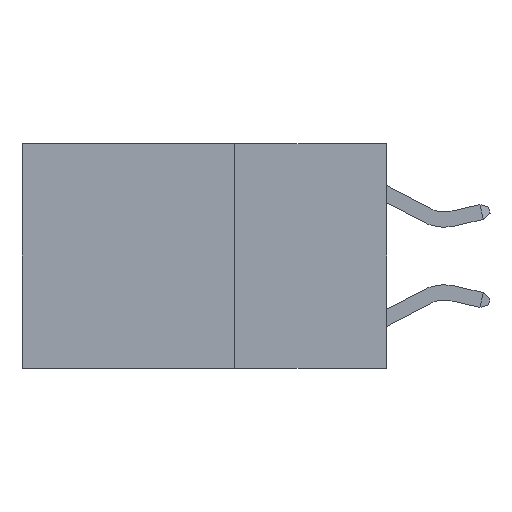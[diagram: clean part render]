
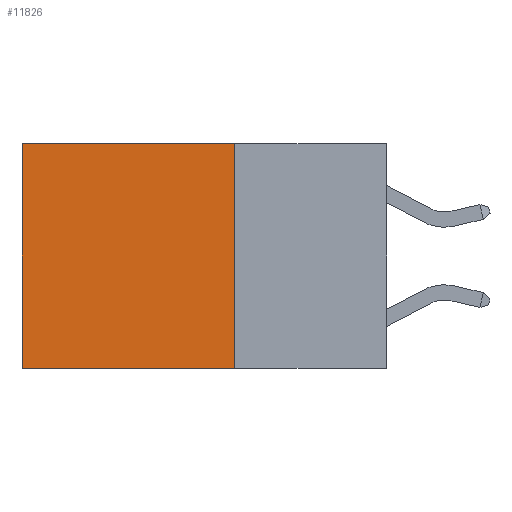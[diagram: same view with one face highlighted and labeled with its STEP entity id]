
A CAD part, left-side view. The second image highlights one B-rep face of the part: STEP entity #11826.
In plain terms, the highlighted planar face has unit normal (-1, 0, 0).
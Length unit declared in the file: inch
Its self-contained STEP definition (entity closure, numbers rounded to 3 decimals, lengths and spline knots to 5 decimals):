
#367 = VECTOR ( 'NONE', #10059, 39.37008 ) ;
#1426 = CARTESIAN_POINT ( 'NONE',  ( 0.2625, 0.25, -0.37 ) ) ;
#1536 = LINE ( 'NONE', #1426, #367 ) ;
#2218 = DIRECTION ( 'NONE',  ( 1., 0., 0. ) ) ;
#2482 = EDGE_CURVE ( 'NONE', #7998, #12967, #1536, .T. ) ;
#2577 = LINE ( 'NONE', #7992, #11697 ) ;
#3062 = FACE_OUTER_BOUND ( 'NONE', #7235, .T. ) ;
#3625 = CARTESIAN_POINT ( 'NONE',  ( 0.2625, 0.25, 0. ) ) ;
#4370 = VERTEX_POINT ( 'NONE', #8994 ) ;
#4670 = ORIENTED_EDGE ( 'NONE', *, *, #5070, .F. ) ;
#5047 = EDGE_CURVE ( 'NONE', #4370, #9518, #8269, .T. ) ;
#5070 = EDGE_CURVE ( 'NONE', #4370, #7998, #2577, .T. ) ;
#5331 = LINE ( 'NONE', #12869, #15397 ) ;
#5552 = DIRECTION ( 'NONE',  ( 0., 0., -1. ) ) ;
#7206 = PLANE ( 'NONE',  #10110 ) ;
#7235 = EDGE_LOOP ( 'NONE', ( #14538, #11356, #4670, #15577 ) ) ;
#7992 = CARTESIAN_POINT ( 'NONE',  ( 0.2625, 0.25, 0. ) ) ;
#7998 = VERTEX_POINT ( 'NONE', #10356 ) ;
#8269 = LINE ( 'NONE', #13014, #9039 ) ;
#8554 = CARTESIAN_POINT ( 'NONE',  ( 0.2625, 0.6, 0. ) ) ;
#8994 = CARTESIAN_POINT ( 'NONE',  ( 0.2625, 0.25, 0. ) ) ;
#9039 = VECTOR ( 'NONE', #15235, 39.37008 ) ;
#9518 = VERTEX_POINT ( 'NONE', #8554 ) ;
#10059 = DIRECTION ( 'NONE',  ( 0., 1., 0. ) ) ;
#10110 = AXIS2_PLACEMENT_3D ( 'NONE', #3625, #2218, #10727 ) ;
#10356 = CARTESIAN_POINT ( 'NONE',  ( 0.2625, 0.25, -0.37 ) ) ;
#10727 = DIRECTION ( 'NONE',  ( 0., 0., -1. ) ) ;
#11356 = ORIENTED_EDGE ( 'NONE', *, *, #2482, .F. ) ;
#11697 = VECTOR ( 'NONE', #13225, 39.37008 ) ;
#11826 = ADVANCED_FACE ( 'NONE', ( #3062 ), #7206, .F. ) ;
#12869 = CARTESIAN_POINT ( 'NONE',  ( 0.2625, 0.6, 0. ) ) ;
#12967 = VERTEX_POINT ( 'NONE', #14759 ) ;
#13014 = CARTESIAN_POINT ( 'NONE',  ( 0.2625, 0.25, 0. ) ) ;
#13225 = DIRECTION ( 'NONE',  ( 0., 0., -1. ) ) ;
#14538 = ORIENTED_EDGE ( 'NONE', *, *, #15135, .T. ) ;
#14759 = CARTESIAN_POINT ( 'NONE',  ( 0.2625, 0.6, -0.37 ) ) ;
#15135 = EDGE_CURVE ( 'NONE', #9518, #12967, #5331, .T. ) ;
#15235 = DIRECTION ( 'NONE',  ( 0., 1., 0. ) ) ;
#15397 = VECTOR ( 'NONE', #5552, 39.37008 ) ;
#15577 = ORIENTED_EDGE ( 'NONE', *, *, #5047, .T. ) ;
